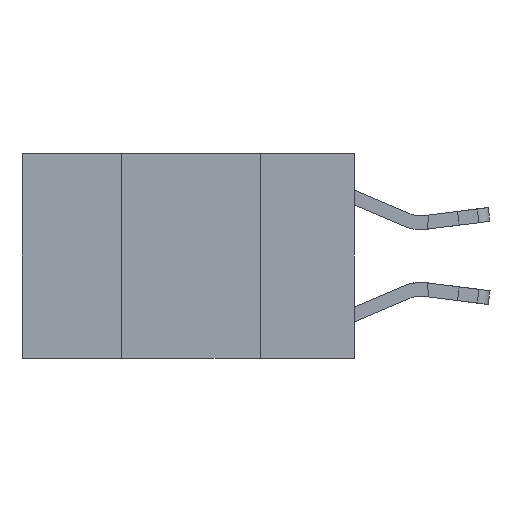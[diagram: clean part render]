
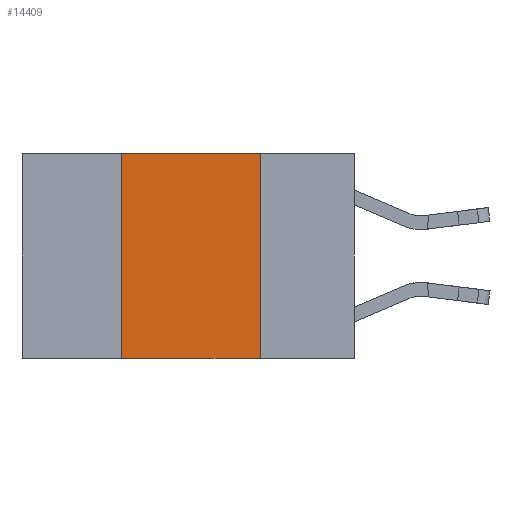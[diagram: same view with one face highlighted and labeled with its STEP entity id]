
A CAD part, left-side view. The second image highlights one B-rep face of the part: STEP entity #14409.
In plain terms, the highlighted planar face has unit normal (-1, 0, 0).
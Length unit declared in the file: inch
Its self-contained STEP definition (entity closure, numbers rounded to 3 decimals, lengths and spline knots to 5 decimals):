
#254 = ORIENTED_EDGE ( 'NONE', *, *, #15758, .F. ) ;
#466 = ORIENTED_EDGE ( 'NONE', *, *, #14406, .T. ) ;
#2252 = CARTESIAN_POINT ( 'NONE',  ( 0., 0.17, -0.37 ) ) ;
#2802 = VERTEX_POINT ( 'NONE', #23874 ) ;
#2939 = CARTESIAN_POINT ( 'NONE',  ( 0., 0.42, 0. ) ) ;
#3384 = VECTOR ( 'NONE', #16203, 39.37008 ) ;
#4365 = LINE ( 'NONE', #16172, #19012 ) ;
#6187 = CARTESIAN_POINT ( 'NONE',  ( 0., 0.6, 0. ) ) ;
#6695 = VECTOR ( 'NONE', #21787, 39.37008 ) ;
#7843 = FACE_OUTER_BOUND ( 'NONE', #19611, .T. ) ;
#8520 = ORIENTED_EDGE ( 'NONE', *, *, #17050, .F. ) ;
#9881 = CARTESIAN_POINT ( 'NONE',  ( 0., 0.6, 0. ) ) ;
#10247 = DIRECTION ( 'NONE',  ( 0., 0., -1. ) ) ;
#11324 = VERTEX_POINT ( 'NONE', #2939 ) ;
#12056 = LINE ( 'NONE', #9881, #6695 ) ;
#13302 = CARTESIAN_POINT ( 'NONE',  ( 0., 0.17, 0. ) ) ;
#14206 = CARTESIAN_POINT ( 'NONE',  ( 0., 0.42, 0. ) ) ;
#14406 = EDGE_CURVE ( 'NONE', #2802, #18440, #4365, .T. ) ;
#14409 = ADVANCED_FACE ( 'NONE', ( #7843 ), #20092, .F. ) ;
#14414 = DIRECTION ( 'NONE',  ( 0., 0., -1. ) ) ;
#15264 = LINE ( 'NONE', #18322, #20459 ) ;
#15758 = EDGE_CURVE ( 'NONE', #2802, #11324, #18940, .T. ) ;
#16172 = CARTESIAN_POINT ( 'NONE',  ( 0., 0.6, -0.37 ) ) ;
#16203 = DIRECTION ( 'NONE',  ( 0., 0., 1. ) ) ;
#17050 = EDGE_CURVE ( 'NONE', #23440, #18440, #15264, .T. ) ;
#17891 = ORIENTED_EDGE ( 'NONE', *, *, #18311, .F. ) ;
#18105 = DIRECTION ( 'NONE',  ( 0., -1., 0. ) ) ;
#18311 = EDGE_CURVE ( 'NONE', #11324, #23440, #12056, .T. ) ;
#18322 = CARTESIAN_POINT ( 'NONE',  ( 0., 0.17, 0. ) ) ;
#18440 = VERTEX_POINT ( 'NONE', #2252 ) ;
#18940 = LINE ( 'NONE', #14206, #3384 ) ;
#19012 = VECTOR ( 'NONE', #18105, 39.37008 ) ;
#19611 = EDGE_LOOP ( 'NONE', ( #8520, #17891, #254, #466 ) ) ;
#19781 = AXIS2_PLACEMENT_3D ( 'NONE', #6187, #22079, #10247 ) ;
#20092 = PLANE ( 'NONE',  #19781 ) ;
#20459 = VECTOR ( 'NONE', #14414, 39.37008 ) ;
#21787 = DIRECTION ( 'NONE',  ( 0., -1., 0. ) ) ;
#22079 = DIRECTION ( 'NONE',  ( 1., 0., 0. ) ) ;
#23440 = VERTEX_POINT ( 'NONE', #13302 ) ;
#23874 = CARTESIAN_POINT ( 'NONE',  ( 0., 0.42, -0.37 ) ) ;
